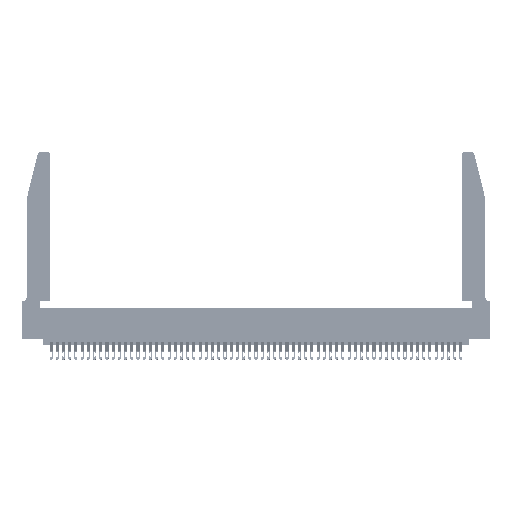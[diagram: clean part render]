
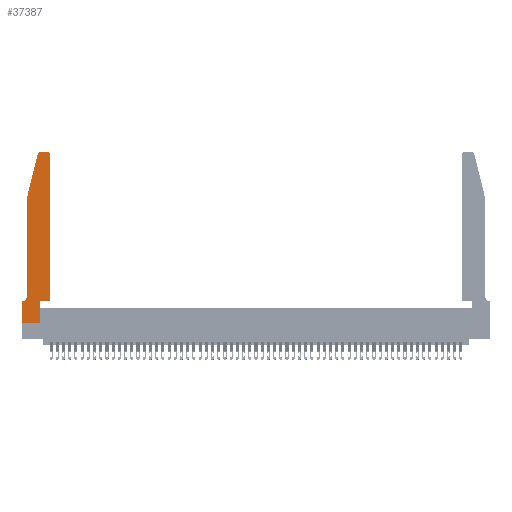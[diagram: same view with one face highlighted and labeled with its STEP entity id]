
A CAD part, top view. The second image highlights one B-rep face of the part: STEP entity #37387.
In plain terms, the highlighted planar face has unit normal (0, 0, 1).
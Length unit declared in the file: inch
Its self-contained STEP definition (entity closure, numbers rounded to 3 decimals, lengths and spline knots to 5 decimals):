
#41 = CARTESIAN_POINT ( 'NONE',  ( 0.284, 2.72, 0.37 ) ) ;
#766 = DIRECTION ( 'NONE',  ( 0., 0., 1. ) ) ;
#934 = VECTOR ( 'NONE', #11049, 39.37008 ) ;
#2725 = DIRECTION ( 'NONE',  ( -1., 0., 0. ) ) ;
#3031 = EDGE_CURVE ( 'NONE', #47543, #22361, #49028, .T. ) ;
#3778 = CARTESIAN_POINT ( 'NONE',  ( 0.0755, 2., 0.37 ) ) ;
#4324 = DIRECTION ( 'NONE',  ( 1., 0., 0. ) ) ;
#4940 = ORIENTED_EDGE ( 'NONE', *, *, #6121, .T. ) ;
#5309 = ORIENTED_EDGE ( 'NONE', *, *, #14575, .T. ) ;
#5456 = VECTOR ( 'NONE', #8047, 39.37008 ) ;
#6121 = EDGE_CURVE ( 'NONE', #23372, #14576, #49919, .T. ) ;
#6822 = LINE ( 'NONE', #3778, #5456 ) ;
#7085 = DIRECTION ( 'NONE',  ( 0., 1., 0. ) ) ;
#7216 = CARTESIAN_POINT ( 'NONE',  ( 0.4505, 0.35, 0.37 ) ) ;
#7327 = CARTESIAN_POINT ( 'NONE',  ( 0.0755, 2., 0.37 ) ) ;
#7597 = VERTEX_POINT ( 'NONE', #28638 ) ;
#7947 = DIRECTION ( 'NONE',  ( 0., 0., -1. ) ) ;
#8047 = DIRECTION ( 'NONE',  ( 0., -1., 0. ) ) ;
#10338 = CARTESIAN_POINT ( 'NONE',  ( 0.4505, 0.35, 0.37 ) ) ;
#11049 = DIRECTION ( 'NONE',  ( 1., 0., 0. ) ) ;
#11329 = CARTESIAN_POINT ( 'NONE',  ( 0.2605, 2.75, 0.37 ) ) ;
#11368 = CARTESIAN_POINT ( 'NONE',  ( 0.0755, 2., 0.37 ) ) ;
#11936 = CARTESIAN_POINT ( 'NONE',  ( 0., 0., 0.37 ) ) ;
#11996 = VERTEX_POINT ( 'NONE', #7216 ) ;
#12124 = CARTESIAN_POINT ( 'NONE',  ( 0.4505, 2.72, 0.37 ) ) ;
#12312 = CARTESIAN_POINT ( 'NONE',  ( 0.0755, 0.42, 0.37 ) ) ;
#12379 = FACE_OUTER_BOUND ( 'NONE', #26347, .T. ) ;
#12391 = AXIS2_PLACEMENT_3D ( 'NONE', #42501, #46688, #21569 ) ;
#13036 = VECTOR ( 'NONE', #7085, 39.37008 ) ;
#14575 = EDGE_CURVE ( 'NONE', #29928, #11996, #43163, .T. ) ;
#14576 = VERTEX_POINT ( 'NONE', #15533 ) ;
#14630 = DIRECTION ( 'NONE',  ( 0., 1., 0. ) ) ;
#15533 = CARTESIAN_POINT ( 'NONE',  ( 0.2865, 0., 0.37 ) ) ;
#16491 = VECTOR ( 'NONE', #27579, 39.37008 ) ;
#16616 = ORIENTED_EDGE ( 'NONE', *, *, #47690, .T. ) ;
#17571 = LINE ( 'NONE', #10338, #38649 ) ;
#18070 = VECTOR ( 'NONE', #32810, 39.37008 ) ;
#18821 = ORIENTED_EDGE ( 'NONE', *, *, #45703, .T. ) ;
#19292 = CARTESIAN_POINT ( 'NONE',  ( 0.25487, 2.72718, 0.37 ) ) ;
#19426 = AXIS2_PLACEMENT_3D ( 'NONE', #26130, #766, #30336 ) ;
#19549 = VERTEX_POINT ( 'NONE', #12312 ) ;
#19559 = CARTESIAN_POINT ( 'NONE',  ( 0.0755, 0.35, 0.37 ) ) ;
#19577 = EDGE_CURVE ( 'NONE', #7597, #38138, #41087, .T. ) ;
#19760 = CARTESIAN_POINT ( 'NONE',  ( 0.4505, 0.35, 0.37 ) ) ;
#19959 = VERTEX_POINT ( 'NONE', #44104 ) ;
#20072 = LINE ( 'NONE', #11329, #50818 ) ;
#21569 = DIRECTION ( 'NONE',  ( 1., 0., 0. ) ) ;
#21993 = CIRCLE ( 'NONE', #19426, 0.03 ) ;
#22079 = CARTESIAN_POINT ( 'NONE',  ( 0.2865, 0.35, 0.37 ) ) ;
#22361 = VERTEX_POINT ( 'NONE', #39198 ) ;
#22704 = ORIENTED_EDGE ( 'NONE', *, *, #53630, .T. ) ;
#23195 = ORIENTED_EDGE ( 'NONE', *, *, #3031, .T. ) ;
#23372 = VERTEX_POINT ( 'NONE', #28312 ) ;
#23917 = CARTESIAN_POINT ( 'NONE',  ( 0.2865, 0.35, 0.37 ) ) ;
#26130 = CARTESIAN_POINT ( 'NONE',  ( 0.4205, 2.72, 0.37 ) ) ;
#26347 = EDGE_LOOP ( 'NONE', ( #35131, #27814, #53344, #31372, #16616, #23195, #22704, #4940, #44352, #5309, #18821, #36054 ) ) ;
#26818 = VECTOR ( 'NONE', #2725, 39.37008 ) ;
#27579 = DIRECTION ( 'NONE',  ( 1., 0., 0. ) ) ;
#27814 = ORIENTED_EDGE ( 'NONE', *, *, #19577, .T. ) ;
#28312 = CARTESIAN_POINT ( 'NONE',  ( 0., 0., 0.37 ) ) ;
#28638 = CARTESIAN_POINT ( 'NONE',  ( 0.284, 2.75, 0.37 ) ) ;
#29295 = LINE ( 'NONE', #7327, #18070 ) ;
#29643 = DIRECTION ( 'NONE',  ( 0., 0., 1. ) ) ;
#29928 = VERTEX_POINT ( 'NONE', #22079 ) ;
#30336 = DIRECTION ( 'NONE',  ( 1., 0., 0. ) ) ;
#31372 = ORIENTED_EDGE ( 'NONE', *, *, #40403, .T. ) ;
#32144 = CARTESIAN_POINT ( 'NONE',  ( 0.0055, 0.35, 0.37 ) ) ;
#32810 = DIRECTION ( 'NONE',  ( -0.239, -0.971, 0. ) ) ;
#33246 = CARTESIAN_POINT ( 'NONE',  ( 0.0055, 0.42, 0.37 ) ) ;
#34095 = PLANE ( 'NONE',  #12391 ) ;
#35131 = ORIENTED_EDGE ( 'NONE', *, *, #46959, .T. ) ;
#35830 = CARTESIAN_POINT ( 'NONE',  ( 0., 0., 0.37 ) ) ;
#36041 = EDGE_CURVE ( 'NONE', #40387, #19959, #21993, .T. ) ;
#36054 = ORIENTED_EDGE ( 'NONE', *, *, #36041, .T. ) ;
#37198 = DIRECTION ( 'NONE',  ( 0., -1., 0. ) ) ;
#37387 = ADVANCED_FACE ( 'NONE', ( #12379 ), #34095, .T. ) ;
#37462 = DIRECTION ( 'NONE',  ( -1., 0., 0. ) ) ;
#38138 = VERTEX_POINT ( 'NONE', #19292 ) ;
#38191 = EDGE_CURVE ( 'NONE', #14576, #29928, #47841, .T. ) ;
#38649 = VECTOR ( 'NONE', #14630, 39.37008 ) ;
#39130 = VECTOR ( 'NONE', #37198, 39.37008 ) ;
#39198 = CARTESIAN_POINT ( 'NONE',  ( 0., 0.35, 0.37 ) ) ;
#40287 = VERTEX_POINT ( 'NONE', #11368 ) ;
#40387 = VERTEX_POINT ( 'NONE', #12124 ) ;
#40403 = EDGE_CURVE ( 'NONE', #40287, #19549, #6822, .T. ) ;
#41087 = CIRCLE ( 'NONE', #48091, 0.03 ) ;
#42501 = CARTESIAN_POINT ( 'NONE',  ( 0., 0.35, 0.37 ) ) ;
#43163 = LINE ( 'NONE', #19760, #934 ) ;
#44104 = CARTESIAN_POINT ( 'NONE',  ( 0.4205, 2.75, 0.37 ) ) ;
#44352 = ORIENTED_EDGE ( 'NONE', *, *, #38191, .T. ) ;
#44793 = AXIS2_PLACEMENT_3D ( 'NONE', #33246, #7947, #37462 ) ;
#45016 = DIRECTION ( 'NONE',  ( -1., 0., 0. ) ) ;
#45703 = EDGE_CURVE ( 'NONE', #11996, #40387, #17571, .T. ) ;
#46688 = DIRECTION ( 'NONE',  ( 0., 0., 1. ) ) ;
#46959 = EDGE_CURVE ( 'NONE', #19959, #7597, #20072, .T. ) ;
#47537 = CIRCLE ( 'NONE', #44793, 0.07 ) ;
#47543 = VERTEX_POINT ( 'NONE', #32144 ) ;
#47690 = EDGE_CURVE ( 'NONE', #19549, #47543, #47537, .T. ) ;
#47841 = LINE ( 'NONE', #23917, #13036 ) ;
#48091 = AXIS2_PLACEMENT_3D ( 'NONE', #41, #29643, #4324 ) ;
#48886 = LINE ( 'NONE', #11936, #39130 ) ;
#49028 = LINE ( 'NONE', #19559, #26818 ) ;
#49919 = LINE ( 'NONE', #35830, #16491 ) ;
#50818 = VECTOR ( 'NONE', #45016, 39.37008 ) ;
#53344 = ORIENTED_EDGE ( 'NONE', *, *, #53573, .T. ) ;
#53573 = EDGE_CURVE ( 'NONE', #38138, #40287, #29295, .T. ) ;
#53630 = EDGE_CURVE ( 'NONE', #22361, #23372, #48886, .T. ) ;
